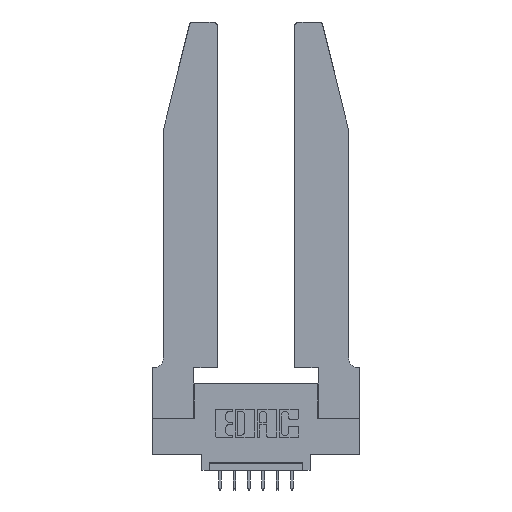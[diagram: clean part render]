
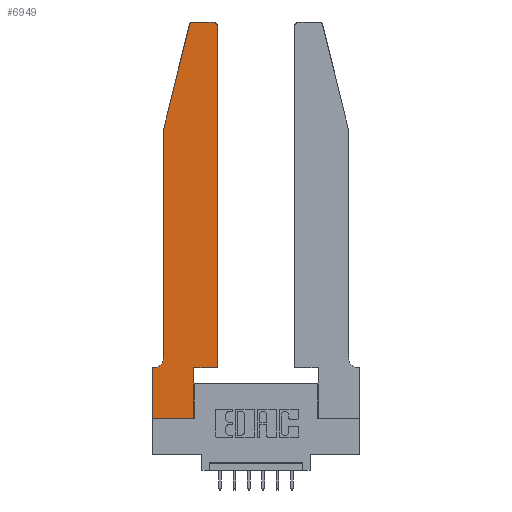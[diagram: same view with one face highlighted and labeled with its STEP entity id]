
A CAD part, top view. The second image highlights one B-rep face of the part: STEP entity #6949.
In plain terms, the highlighted planar face has unit normal (0, 0, 1).
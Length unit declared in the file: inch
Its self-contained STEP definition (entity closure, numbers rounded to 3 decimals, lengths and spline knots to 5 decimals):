
#331 = DIRECTION ( 'NONE',  ( -0.239, -0.971, 0. ) ) ;
#379 = VERTEX_POINT ( 'NONE', #12256 ) ;
#476 = VECTOR ( 'NONE', #1883, 39.37008 ) ;
#581 = VERTEX_POINT ( 'NONE', #12686 ) ;
#619 = CARTESIAN_POINT ( 'NONE',  ( 0.0755, 2., 0.37 ) ) ;
#620 = VERTEX_POINT ( 'NONE', #10390 ) ;
#766 = DIRECTION ( 'NONE',  ( 0., 1., 0. ) ) ;
#877 = DIRECTION ( 'NONE',  ( 0., 0., -1. ) ) ;
#913 = CARTESIAN_POINT ( 'NONE',  ( 0.4205, 2.75, 0.37 ) ) ;
#1067 = CARTESIAN_POINT ( 'NONE',  ( 0.284, 2.72, 0.37 ) ) ;
#1070 = VECTOR ( 'NONE', #4619, 39.37008 ) ;
#1432 = CARTESIAN_POINT ( 'NONE',  ( 0.2605, 2.75, 0.37 ) ) ;
#1457 = ORIENTED_EDGE ( 'NONE', *, *, #5734, .T. ) ;
#1653 = LINE ( 'NONE', #12676, #6919 ) ;
#1704 = VECTOR ( 'NONE', #4400, 39.37008 ) ;
#1757 = VECTOR ( 'NONE', #11665, 39.37008 ) ;
#1883 = DIRECTION ( 'NONE',  ( 0., -1., 0. ) ) ;
#1889 = DIRECTION ( 'NONE',  ( -1., 0., 0. ) ) ;
#2060 = VERTEX_POINT ( 'NONE', #913 ) ;
#2204 = AXIS2_PLACEMENT_3D ( 'NONE', #10625, #877, #1889 ) ;
#2215 = VERTEX_POINT ( 'NONE', #6932 ) ;
#2307 = ORIENTED_EDGE ( 'NONE', *, *, #6441, .T. ) ;
#2358 = DIRECTION ( 'NONE',  ( 1., 0., 0. ) ) ;
#2433 = AXIS2_PLACEMENT_3D ( 'NONE', #1067, #10010, #10216 ) ;
#2762 = DIRECTION ( 'NONE',  ( 0., 0., 1. ) ) ;
#2834 = VERTEX_POINT ( 'NONE', #11424 ) ;
#3213 = EDGE_CURVE ( 'NONE', #2834, #13335, #10595, .T. ) ;
#3245 = VECTOR ( 'NONE', #10087, 39.37008 ) ;
#4032 = VERTEX_POINT ( 'NONE', #4353 ) ;
#4072 = VERTEX_POINT ( 'NONE', #5070 ) ;
#4175 = CIRCLE ( 'NONE', #6025, 0.03 ) ;
#4238 = EDGE_CURVE ( 'NONE', #4072, #2834, #14329, .T. ) ;
#4353 = CARTESIAN_POINT ( 'NONE',  ( 0.4505, 0.35, 0.37 ) ) ;
#4400 = DIRECTION ( 'NONE',  ( 0., -1., 0. ) ) ;
#4405 = ORIENTED_EDGE ( 'NONE', *, *, #13688, .T. ) ;
#4483 = ORIENTED_EDGE ( 'NONE', *, *, #11919, .T. ) ;
#4619 = DIRECTION ( 'NONE',  ( 1., 0., 0. ) ) ;
#5070 = CARTESIAN_POINT ( 'NONE',  ( 0., 0.35, 0.37 ) ) ;
#5152 = DIRECTION ( 'NONE',  ( 1., 0., 0. ) ) ;
#5298 = CARTESIAN_POINT ( 'NONE',  ( 0.2865, 0., 0.37 ) ) ;
#5367 = EDGE_CURVE ( 'NONE', #581, #379, #6597, .T. ) ;
#5565 = EDGE_CURVE ( 'NONE', #379, #10782, #6141, .T. ) ;
#5668 = ORIENTED_EDGE ( 'NONE', *, *, #4238, .T. ) ;
#5734 = EDGE_CURVE ( 'NONE', #13335, #620, #13082, .T. ) ;
#5921 = CARTESIAN_POINT ( 'NONE',  ( 0.0755, 0.42, 0.37 ) ) ;
#5923 = AXIS2_PLACEMENT_3D ( 'NONE', #10061, #6712, #2358 ) ;
#6025 = AXIS2_PLACEMENT_3D ( 'NONE', #7183, #2762, #5152 ) ;
#6141 = LINE ( 'NONE', #619, #9151 ) ;
#6413 = ORIENTED_EDGE ( 'NONE', *, *, #5367, .T. ) ;
#6441 = EDGE_CURVE ( 'NONE', #9265, #2215, #12864, .T. ) ;
#6595 = ORIENTED_EDGE ( 'NONE', *, *, #6733, .T. ) ;
#6597 = CIRCLE ( 'NONE', #2433, 0.03 ) ;
#6712 = DIRECTION ( 'NONE',  ( 0., 0., 1. ) ) ;
#6733 = EDGE_CURVE ( 'NONE', #2215, #4072, #7231, .T. ) ;
#6919 = VECTOR ( 'NONE', #11536, 39.37008 ) ;
#6932 = CARTESIAN_POINT ( 'NONE',  ( 0.0055, 0.35, 0.37 ) ) ;
#6949 = ADVANCED_FACE ( 'NONE', ( #11006 ), #13377, .T. ) ;
#7183 = CARTESIAN_POINT ( 'NONE',  ( 0.4205, 2.72, 0.37 ) ) ;
#7231 = LINE ( 'NONE', #9501, #1757 ) ;
#7250 = VECTOR ( 'NONE', #8327, 39.37008 ) ;
#7425 = CARTESIAN_POINT ( 'NONE',  ( 0.4505, 2.72, 0.37 ) ) ;
#7507 = CARTESIAN_POINT ( 'NONE',  ( 0.2865, 0.35, 0.37 ) ) ;
#7734 = CARTESIAN_POINT ( 'NONE',  ( 0., 0., 0.37 ) ) ;
#8007 = VERTEX_POINT ( 'NONE', #7425 ) ;
#8065 = ORIENTED_EDGE ( 'NONE', *, *, #9085, .T. ) ;
#8327 = DIRECTION ( 'NONE',  ( 1., 0., 0. ) ) ;
#8471 = CARTESIAN_POINT ( 'NONE',  ( 0., 0., 0.37 ) ) ;
#8984 = LINE ( 'NONE', #9126, #1070 ) ;
#9085 = EDGE_CURVE ( 'NONE', #620, #4032, #8984, .T. ) ;
#9126 = CARTESIAN_POINT ( 'NONE',  ( 0.4505, 0.35, 0.37 ) ) ;
#9151 = VECTOR ( 'NONE', #331, 39.37008 ) ;
#9265 = VERTEX_POINT ( 'NONE', #5921 ) ;
#9377 = EDGE_LOOP ( 'NONE', ( #14309, #6413, #10868, #13209, #2307, #6595, #5668, #12319, #1457, #8065, #4405, #4483 ) ) ;
#9501 = CARTESIAN_POINT ( 'NONE',  ( 0.0755, 0.35, 0.37 ) ) ;
#10010 = DIRECTION ( 'NONE',  ( 0., 0., 1. ) ) ;
#10061 = CARTESIAN_POINT ( 'NONE',  ( 0., 0.35, 0.37 ) ) ;
#10087 = DIRECTION ( 'NONE',  ( -1., 0., 0. ) ) ;
#10216 = DIRECTION ( 'NONE',  ( 1., 0., 0. ) ) ;
#10390 = CARTESIAN_POINT ( 'NONE',  ( 0.2865, 0.35, 0.37 ) ) ;
#10595 = LINE ( 'NONE', #8471, #7250 ) ;
#10625 = CARTESIAN_POINT ( 'NONE',  ( 0.0055, 0.42, 0.37 ) ) ;
#10782 = VERTEX_POINT ( 'NONE', #13147 ) ;
#10827 = CARTESIAN_POINT ( 'NONE',  ( 0.0755, 2., 0.37 ) ) ;
#10868 = ORIENTED_EDGE ( 'NONE', *, *, #5565, .T. ) ;
#11006 = FACE_OUTER_BOUND ( 'NONE', #9377, .T. ) ;
#11392 = LINE ( 'NONE', #1432, #3245 ) ;
#11424 = CARTESIAN_POINT ( 'NONE',  ( 0., 0., 0.37 ) ) ;
#11536 = DIRECTION ( 'NONE',  ( 0., 1., 0. ) ) ;
#11665 = DIRECTION ( 'NONE',  ( -1., 0., 0. ) ) ;
#11919 = EDGE_CURVE ( 'NONE', #8007, #2060, #4175, .T. ) ;
#12078 = EDGE_CURVE ( 'NONE', #10782, #9265, #14205, .T. ) ;
#12226 = EDGE_CURVE ( 'NONE', #2060, #581, #11392, .T. ) ;
#12256 = CARTESIAN_POINT ( 'NONE',  ( 0.25487, 2.72718, 0.37 ) ) ;
#12319 = ORIENTED_EDGE ( 'NONE', *, *, #3213, .T. ) ;
#12676 = CARTESIAN_POINT ( 'NONE',  ( 0.4505, 0.35, 0.37 ) ) ;
#12686 = CARTESIAN_POINT ( 'NONE',  ( 0.284, 2.75, 0.37 ) ) ;
#12864 = CIRCLE ( 'NONE', #2204, 0.07 ) ;
#13082 = LINE ( 'NONE', #7507, #14233 ) ;
#13147 = CARTESIAN_POINT ( 'NONE',  ( 0.0755, 2., 0.37 ) ) ;
#13209 = ORIENTED_EDGE ( 'NONE', *, *, #12078, .T. ) ;
#13335 = VERTEX_POINT ( 'NONE', #5298 ) ;
#13377 = PLANE ( 'NONE',  #5923 ) ;
#13688 = EDGE_CURVE ( 'NONE', #4032, #8007, #1653, .T. ) ;
#14205 = LINE ( 'NONE', #10827, #476 ) ;
#14233 = VECTOR ( 'NONE', #766, 39.37008 ) ;
#14309 = ORIENTED_EDGE ( 'NONE', *, *, #12226, .T. ) ;
#14329 = LINE ( 'NONE', #7734, #1704 ) ;
